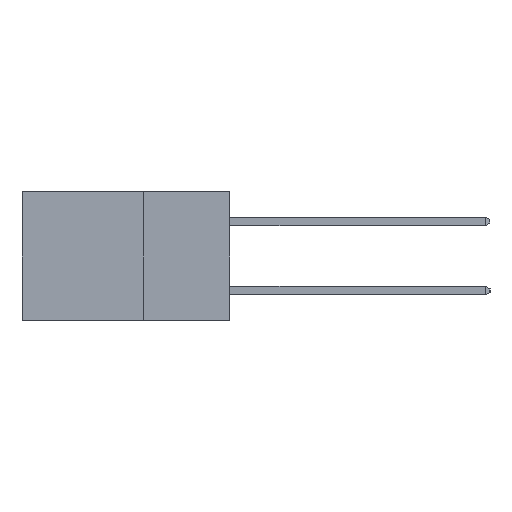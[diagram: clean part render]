
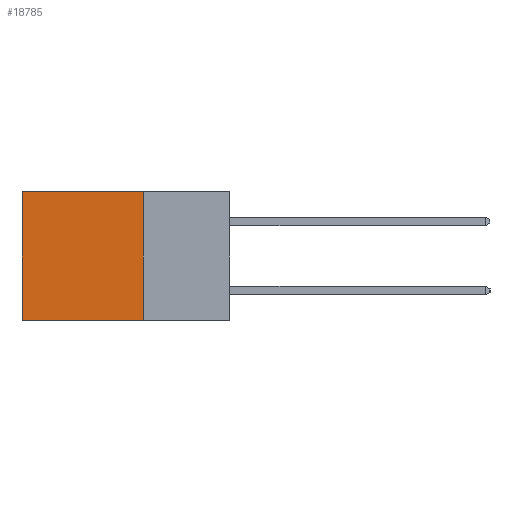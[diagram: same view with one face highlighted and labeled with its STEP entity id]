
A CAD part, left-side view. The second image highlights one B-rep face of the part: STEP entity #18785.
In plain terms, the highlighted planar face has unit normal (-1, 0, 0).
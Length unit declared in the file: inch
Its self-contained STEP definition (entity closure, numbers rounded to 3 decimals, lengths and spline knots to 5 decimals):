
#26 = LINE ( 'NONE', #3673, #20818 ) ;
#2179 = ORIENTED_EDGE ( 'NONE', *, *, #20285, .T. ) ;
#3086 = DIRECTION ( 'NONE',  ( 0., 1., 0. ) ) ;
#3156 = VECTOR ( 'NONE', #3086, 39.37008 ) ;
#3673 = CARTESIAN_POINT ( 'NONE',  ( 0.2615, 0.25, -0.37 ) ) ;
#4369 = ORIENTED_EDGE ( 'NONE', *, *, #13531, .F. ) ;
#5067 = CARTESIAN_POINT ( 'NONE',  ( 0.2615, 0.25, -0.37 ) ) ;
#5785 = PLANE ( 'NONE',  #22040 ) ;
#7366 = EDGE_CURVE ( 'NONE', #24018, #19491, #26, .T. ) ;
#8018 = CARTESIAN_POINT ( 'NONE',  ( 0.2615, 0.25, 0. ) ) ;
#8293 = LINE ( 'NONE', #13586, #23064 ) ;
#9508 = ORIENTED_EDGE ( 'NONE', *, *, #24305, .T. ) ;
#9850 = LINE ( 'NONE', #5067, #3156 ) ;
#9856 = DIRECTION ( 'NONE',  ( 0., 0., -1. ) ) ;
#10472 = ORIENTED_EDGE ( 'NONE', *, *, #7366, .F. ) ;
#11681 = CARTESIAN_POINT ( 'NONE',  ( 0.2615, 0.25, -0.37 ) ) ;
#11841 = DIRECTION ( 'NONE',  ( 0., 0., -1. ) ) ;
#12640 = CARTESIAN_POINT ( 'NONE',  ( 0.2615, 0.25, 0. ) ) ;
#13531 = EDGE_CURVE ( 'NONE', #19491, #19666, #9850, .T. ) ;
#13586 = CARTESIAN_POINT ( 'NONE',  ( 0.2615, 0.6, -0.37 ) ) ;
#17524 = VERTEX_POINT ( 'NONE', #25441 ) ;
#17608 = FACE_OUTER_BOUND ( 'NONE', #25119, .T. ) ;
#18457 = VECTOR ( 'NONE', #20053, 39.37008 ) ;
#18785 = ADVANCED_FACE ( 'NONE', ( #17608 ), #5785, .F. ) ;
#19491 = VERTEX_POINT ( 'NONE', #11681 ) ;
#19666 = VERTEX_POINT ( 'NONE', #20256 ) ;
#19852 = CARTESIAN_POINT ( 'NONE',  ( 0.2615, 0.25, -0.37 ) ) ;
#20053 = DIRECTION ( 'NONE',  ( 0., 1., 0. ) ) ;
#20256 = CARTESIAN_POINT ( 'NONE',  ( 0.2615, 0.6, -0.37 ) ) ;
#20285 = EDGE_CURVE ( 'NONE', #24018, #17524, #23784, .T. ) ;
#20818 = VECTOR ( 'NONE', #11841, 39.37008 ) ;
#21876 = DIRECTION ( 'NONE',  ( 1., 0., 0. ) ) ;
#22040 = AXIS2_PLACEMENT_3D ( 'NONE', #19852, #21876, #9856 ) ;
#23064 = VECTOR ( 'NONE', #25513, 39.37008 ) ;
#23784 = LINE ( 'NONE', #8018, #18457 ) ;
#24018 = VERTEX_POINT ( 'NONE', #12640 ) ;
#24305 = EDGE_CURVE ( 'NONE', #17524, #19666, #8293, .T. ) ;
#25119 = EDGE_LOOP ( 'NONE', ( #9508, #4369, #10472, #2179 ) ) ;
#25441 = CARTESIAN_POINT ( 'NONE',  ( 0.2615, 0.6, 0. ) ) ;
#25513 = DIRECTION ( 'NONE',  ( 0., 0., -1. ) ) ;
